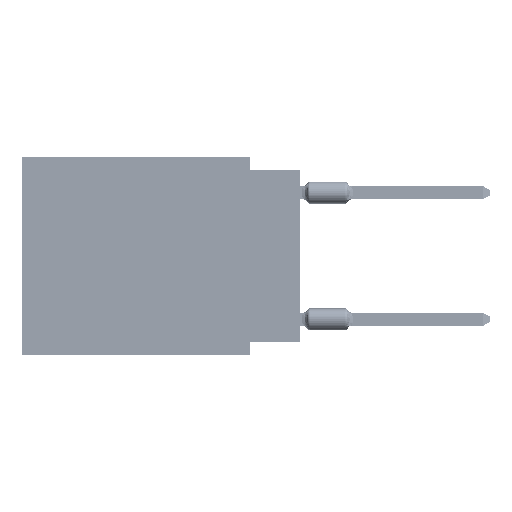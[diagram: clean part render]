
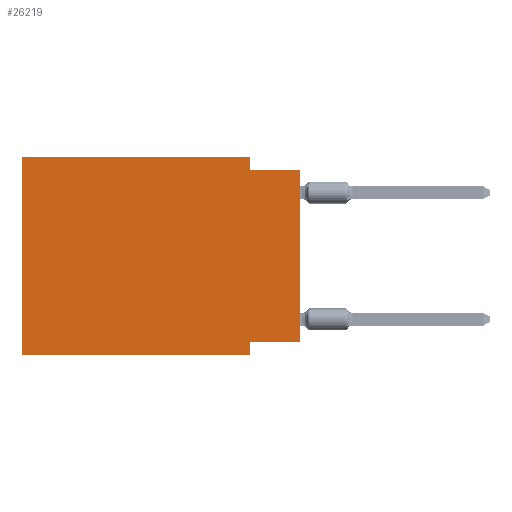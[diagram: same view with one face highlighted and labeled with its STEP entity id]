
A CAD part, left-side view. The second image highlights one B-rep face of the part: STEP entity #26219.
In plain terms, the highlighted planar face has unit normal (-1, 0, 0).
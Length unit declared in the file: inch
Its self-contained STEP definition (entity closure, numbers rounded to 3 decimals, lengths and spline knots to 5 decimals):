
#1743 = CARTESIAN_POINT ( 'NONE',  ( 0., 0., -0.365 ) ) ;
#2502 = CARTESIAN_POINT ( 'NONE',  ( 0., 0.1, 0. ) ) ;
#3214 = VECTOR ( 'NONE', #16772, 39.37008 ) ;
#3286 = VERTEX_POINT ( 'NONE', #71873 ) ;
#4743 = VERTEX_POINT ( 'NONE', #6297 ) ;
#4905 = EDGE_CURVE ( 'NONE', #29857, #35766, #65505, .T. ) ;
#6297 = CARTESIAN_POINT ( 'NONE',  ( 0., 0.1, -0.39 ) ) ;
#6764 = AXIS2_PLACEMENT_3D ( 'NONE', #19788, #65693, #14957 ) ;
#7307 = DIRECTION ( 'NONE',  ( 0., 1., 0. ) ) ;
#7406 = DIRECTION ( 'NONE',  ( 0., -1., 0. ) ) ;
#8881 = EDGE_LOOP ( 'NONE', ( #63623, #49039, #56602, #65470, #50070, #33177, #62952, #47244 ) ) ;
#11285 = CARTESIAN_POINT ( 'NONE',  ( 0., 0., -0.365 ) ) ;
#12671 = VERTEX_POINT ( 'NONE', #19995 ) ;
#13175 = VECTOR ( 'NONE', #7307, 39.37008 ) ;
#13346 = LINE ( 'NONE', #35916, #44436 ) ;
#13665 = LINE ( 'NONE', #58484, #65695 ) ;
#14079 = CARTESIAN_POINT ( 'NONE',  ( 0., 0., -0.025 ) ) ;
#14957 = DIRECTION ( 'NONE',  ( 0., 0., -1. ) ) ;
#15123 = DIRECTION ( 'NONE',  ( 0., 0., 1. ) ) ;
#15930 = CARTESIAN_POINT ( 'NONE',  ( 0., 0.1, -0.365 ) ) ;
#16687 = LINE ( 'NONE', #55949, #54024 ) ;
#16772 = DIRECTION ( 'NONE',  ( 0., -1., 0. ) ) ;
#17991 = VECTOR ( 'NONE', #20230, 39.37008 ) ;
#19788 = CARTESIAN_POINT ( 'NONE',  ( 0., 0.55, 0. ) ) ;
#19995 = CARTESIAN_POINT ( 'NONE',  ( 0., 0.55, 0. ) ) ;
#20230 = DIRECTION ( 'NONE',  ( 0., -1., 0. ) ) ;
#20509 = PLANE ( 'NONE',  #6764 ) ;
#24035 = DIRECTION ( 'NONE',  ( 0., 0., -1. ) ) ;
#24819 = EDGE_CURVE ( 'NONE', #3286, #4743, #13346, .T. ) ;
#26219 = ADVANCED_FACE ( 'NONE', ( #60147 ), #20509, .F. ) ;
#26316 = EDGE_CURVE ( 'NONE', #12671, #40736, #43814, .T. ) ;
#27067 = DIRECTION ( 'NONE',  ( 0., 0., -1. ) ) ;
#28072 = EDGE_CURVE ( 'NONE', #40736, #70328, #16687, .T. ) ;
#29857 = VERTEX_POINT ( 'NONE', #11285 ) ;
#31905 = CARTESIAN_POINT ( 'NONE',  ( 0., 0.55, 0. ) ) ;
#32987 = VERTEX_POINT ( 'NONE', #15930 ) ;
#33177 = ORIENTED_EDGE ( 'NONE', *, *, #24819, .T. ) ;
#34140 = EDGE_CURVE ( 'NONE', #3286, #12671, #72268, .T. ) ;
#34868 = EDGE_CURVE ( 'NONE', #29857, #32987, #52116, .T. ) ;
#35766 = VERTEX_POINT ( 'NONE', #14079 ) ;
#35916 = CARTESIAN_POINT ( 'NONE',  ( 0., 0.55, -0.39 ) ) ;
#40736 = VERTEX_POINT ( 'NONE', #2502 ) ;
#41722 = CARTESIAN_POINT ( 'NONE',  ( 0., 0., -0.025 ) ) ;
#43156 = EDGE_CURVE ( 'NONE', #32987, #4743, #13665, .T. ) ;
#43814 = LINE ( 'NONE', #66414, #3214 ) ;
#44436 = VECTOR ( 'NONE', #7406, 39.37008 ) ;
#47244 = ORIENTED_EDGE ( 'NONE', *, *, #34868, .F. ) ;
#47641 = VECTOR ( 'NONE', #15123, 39.37008 ) ;
#49039 = ORIENTED_EDGE ( 'NONE', *, *, #59154, .F. ) ;
#49167 = CARTESIAN_POINT ( 'NONE',  ( 0., 0., 0. ) ) ;
#49584 = CARTESIAN_POINT ( 'NONE',  ( 0., 0.1, -0.025 ) ) ;
#50003 = DIRECTION ( 'NONE',  ( 0., 0., 1. ) ) ;
#50070 = ORIENTED_EDGE ( 'NONE', *, *, #34140, .F. ) ;
#52111 = VECTOR ( 'NONE', #50003, 39.37008 ) ;
#52116 = LINE ( 'NONE', #1743, #13175 ) ;
#54024 = VECTOR ( 'NONE', #27067, 39.37008 ) ;
#55949 = CARTESIAN_POINT ( 'NONE',  ( 0., 0.1, 0. ) ) ;
#56602 = ORIENTED_EDGE ( 'NONE', *, *, #28072, .F. ) ;
#58484 = CARTESIAN_POINT ( 'NONE',  ( 0., 0.1, -0.39 ) ) ;
#59154 = EDGE_CURVE ( 'NONE', #70328, #35766, #59498, .T. ) ;
#59498 = LINE ( 'NONE', #41722, #17991 ) ;
#60147 = FACE_OUTER_BOUND ( 'NONE', #8881, .T. ) ;
#62952 = ORIENTED_EDGE ( 'NONE', *, *, #43156, .F. ) ;
#63623 = ORIENTED_EDGE ( 'NONE', *, *, #4905, .T. ) ;
#65470 = ORIENTED_EDGE ( 'NONE', *, *, #26316, .F. ) ;
#65505 = LINE ( 'NONE', #49167, #47641 ) ;
#65693 = DIRECTION ( 'NONE',  ( 1., 0., 0. ) ) ;
#65695 = VECTOR ( 'NONE', #24035, 39.37008 ) ;
#66414 = CARTESIAN_POINT ( 'NONE',  ( 0., 0.55, 0. ) ) ;
#70328 = VERTEX_POINT ( 'NONE', #49584 ) ;
#71873 = CARTESIAN_POINT ( 'NONE',  ( 0., 0.55, -0.39 ) ) ;
#72268 = LINE ( 'NONE', #31905, #52111 ) ;
